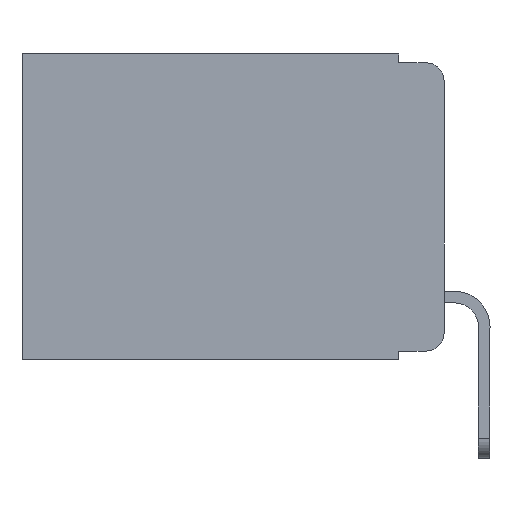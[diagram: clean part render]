
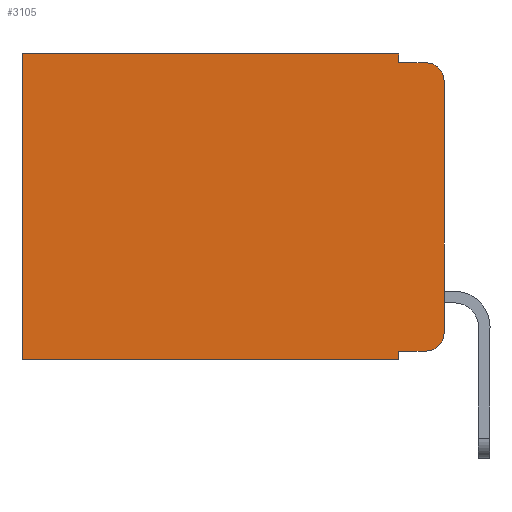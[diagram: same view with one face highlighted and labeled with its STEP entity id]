
A CAD part, left-side view. The second image highlights one B-rep face of the part: STEP entity #3105.
In plain terms, the highlighted planar face has unit normal (-1, 0, 0).
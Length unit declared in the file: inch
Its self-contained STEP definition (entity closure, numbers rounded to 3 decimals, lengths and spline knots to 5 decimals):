
#162 = DIRECTION ( 'NONE',  ( -1., 0., 0. ) ) ;
#246 = ORIENTED_EDGE ( 'NONE', *, *, #6964, .T. ) ;
#349 = EDGE_CURVE ( 'NONE', #9969, #5638, #9700, .T. ) ;
#406 = VECTOR ( 'NONE', #3429, 39.37008 ) ;
#617 = PLANE ( 'NONE',  #1712 ) ;
#720 = LINE ( 'NONE', #4304, #406 ) ;
#971 = DIRECTION ( 'NONE',  ( 0., 0., -1. ) ) ;
#1132 = VECTOR ( 'NONE', #6557, 39.37008 ) ;
#1208 = LINE ( 'NONE', #2872, #1132 ) ;
#1289 = ORIENTED_EDGE ( 'NONE', *, *, #7610, .F. ) ;
#1332 = EDGE_CURVE ( 'NONE', #5638, #3674, #7823, .T. ) ;
#1386 = CIRCLE ( 'NONE', #9469, 0.02 ) ;
#1528 = DIRECTION ( 'NONE',  ( -1., 0., 0. ) ) ;
#1712 = AXIS2_PLACEMENT_3D ( 'NONE', #4205, #7779, #8535 ) ;
#1827 = DIRECTION ( 'NONE',  ( 0., 1., 0. ) ) ;
#1871 = VECTOR ( 'NONE', #1827, 39.37008 ) ;
#2022 = CARTESIAN_POINT ( 'NONE',  ( 0.298, 0., -0.343 ) ) ;
#2230 = CARTESIAN_POINT ( 'NONE',  ( 0.298, 0.473, 0. ) ) ;
#2331 = LINE ( 'NONE', #8069, #10857 ) ;
#2405 = VERTEX_POINT ( 'NONE', #7059 ) ;
#2496 = CARTESIAN_POINT ( 'NONE',  ( 0.298, 0.473, -0.343 ) ) ;
#2872 = CARTESIAN_POINT ( 'NONE',  ( 0.298, 0., 0. ) ) ;
#2961 = CARTESIAN_POINT ( 'NONE',  ( 0.298, 0.051, -0.343 ) ) ;
#2981 = EDGE_CURVE ( 'NONE', #2405, #3674, #1208, .T. ) ;
#3076 = LINE ( 'NONE', #2022, #6353 ) ;
#3105 = ADVANCED_FACE ( 'NONE', ( #11341 ), #617, .F. ) ;
#3429 = DIRECTION ( 'NONE',  ( 0., -1., 0. ) ) ;
#3481 = CARTESIAN_POINT ( 'NONE',  ( 0.298, 0., -0.313 ) ) ;
#3662 = VECTOR ( 'NONE', #9763, 39.37008 ) ;
#3674 = VERTEX_POINT ( 'NONE', #3481 ) ;
#3760 = DIRECTION ( 'NONE',  ( 0., 0., -1. ) ) ;
#3967 = CARTESIAN_POINT ( 'NONE',  ( 0.298, 0.051, 0. ) ) ;
#4205 = CARTESIAN_POINT ( 'NONE',  ( 0.298, 0., 0. ) ) ;
#4304 = CARTESIAN_POINT ( 'NONE',  ( 0.298, 0.051, -0.01 ) ) ;
#4533 = CARTESIAN_POINT ( 'NONE',  ( 0.298, 0., 0. ) ) ;
#4631 = VERTEX_POINT ( 'NONE', #2961 ) ;
#4676 = DIRECTION ( 'NONE',  ( 0., 0., -1. ) ) ;
#4751 = VECTOR ( 'NONE', #4676, 39.37008 ) ;
#4754 = VERTEX_POINT ( 'NONE', #3967 ) ;
#4763 = EDGE_CURVE ( 'NONE', #4754, #7095, #4900, .T. ) ;
#4900 = LINE ( 'NONE', #6431, #4751 ) ;
#4955 = EDGE_CURVE ( 'NONE', #7095, #11247, #720, .T. ) ;
#5580 = CARTESIAN_POINT ( 'NONE',  ( 0.298, 0.02, -0.01 ) ) ;
#5638 = VERTEX_POINT ( 'NONE', #9516 ) ;
#5659 = DIRECTION ( 'NONE',  ( 0., 1., 0. ) ) ;
#5845 = ORIENTED_EDGE ( 'NONE', *, *, #349, .T. ) ;
#6029 = ORIENTED_EDGE ( 'NONE', *, *, #6624, .T. ) ;
#6283 = CARTESIAN_POINT ( 'NONE',  ( 0.298, 0.051, -0.333 ) ) ;
#6312 = ORIENTED_EDGE ( 'NONE', *, *, #1332, .T. ) ;
#6353 = VECTOR ( 'NONE', #5659, 39.37008 ) ;
#6410 = ORIENTED_EDGE ( 'NONE', *, *, #4763, .F. ) ;
#6431 = CARTESIAN_POINT ( 'NONE',  ( 0.298, 0.051, 0. ) ) ;
#6557 = DIRECTION ( 'NONE',  ( 0., 0., -1. ) ) ;
#6624 = EDGE_CURVE ( 'NONE', #8525, #11140, #11548, .T. ) ;
#6806 = ORIENTED_EDGE ( 'NONE', *, *, #2981, .F. ) ;
#6809 = ORIENTED_EDGE ( 'NONE', *, *, #7409, .F. ) ;
#6964 = EDGE_CURVE ( 'NONE', #2405, #11247, #1386, .T. ) ;
#7059 = CARTESIAN_POINT ( 'NONE',  ( 0.298, 0., -0.03 ) ) ;
#7095 = VERTEX_POINT ( 'NONE', #7162 ) ;
#7162 = CARTESIAN_POINT ( 'NONE',  ( 0.298, 0.051, -0.01 ) ) ;
#7356 = ORIENTED_EDGE ( 'NONE', *, *, #9997, .T. ) ;
#7409 = EDGE_CURVE ( 'NONE', #9969, #4631, #2331, .T. ) ;
#7455 = AXIS2_PLACEMENT_3D ( 'NONE', #8205, #162, #3760 ) ;
#7610 = EDGE_CURVE ( 'NONE', #4631, #11140, #3076, .T. ) ;
#7623 = CARTESIAN_POINT ( 'NONE',  ( 0.298, 0.02, -0.03 ) ) ;
#7779 = DIRECTION ( 'NONE',  ( 1., 0., 0. ) ) ;
#7823 = CIRCLE ( 'NONE', #7455, 0.02 ) ;
#7878 = DIRECTION ( 'NONE',  ( 0., 0., -1. ) ) ;
#7981 = CARTESIAN_POINT ( 'NONE',  ( 0.298, 0.051, -0.333 ) ) ;
#7988 = CARTESIAN_POINT ( 'NONE',  ( 0.298, 0.473, 0. ) ) ;
#8069 = CARTESIAN_POINT ( 'NONE',  ( 0.298, 0.051, 0. ) ) ;
#8194 = VECTOR ( 'NONE', #7878, 39.37008 ) ;
#8205 = CARTESIAN_POINT ( 'NONE',  ( 0.298, 0.02, -0.313 ) ) ;
#8525 = VERTEX_POINT ( 'NONE', #2230 ) ;
#8535 = DIRECTION ( 'NONE',  ( 0., 0., -1. ) ) ;
#8683 = DIRECTION ( 'NONE',  ( 0., 0., -1. ) ) ;
#9469 = AXIS2_PLACEMENT_3D ( 'NONE', #7623, #1528, #8683 ) ;
#9516 = CARTESIAN_POINT ( 'NONE',  ( 0.298, 0.02, -0.333 ) ) ;
#9537 = EDGE_LOOP ( 'NONE', ( #6806, #246, #9949, #6410, #7356, #6029, #1289, #6809, #5845, #6312 ) ) ;
#9700 = LINE ( 'NONE', #6283, #3662 ) ;
#9763 = DIRECTION ( 'NONE',  ( 0., -1., 0. ) ) ;
#9949 = ORIENTED_EDGE ( 'NONE', *, *, #4955, .F. ) ;
#9969 = VERTEX_POINT ( 'NONE', #7981 ) ;
#9997 = EDGE_CURVE ( 'NONE', #4754, #8525, #10829, .T. ) ;
#10829 = LINE ( 'NONE', #4533, #1871 ) ;
#10857 = VECTOR ( 'NONE', #971, 39.37008 ) ;
#11140 = VERTEX_POINT ( 'NONE', #2496 ) ;
#11247 = VERTEX_POINT ( 'NONE', #5580 ) ;
#11341 = FACE_OUTER_BOUND ( 'NONE', #9537, .T. ) ;
#11548 = LINE ( 'NONE', #7988, #8194 ) ;
